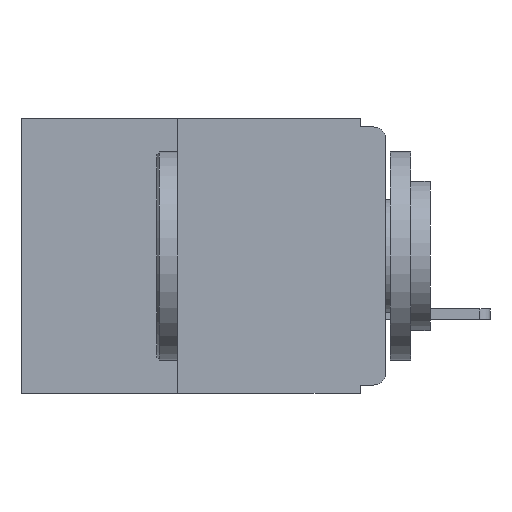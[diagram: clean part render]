
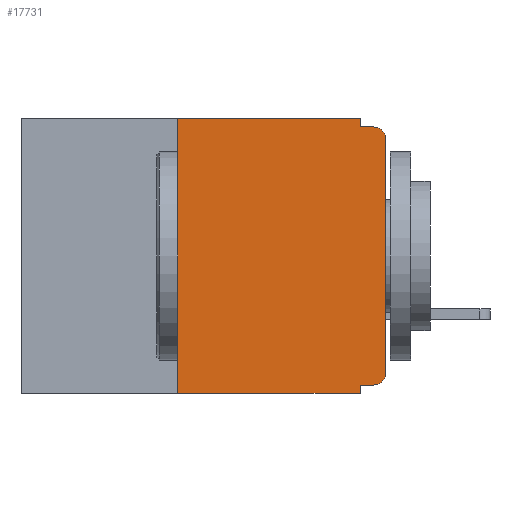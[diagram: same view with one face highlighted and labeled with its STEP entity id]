
A CAD part, left-side view. The second image highlights one B-rep face of the part: STEP entity #17731.
In plain terms, the highlighted planar face has unit normal (-1, 0, 0).
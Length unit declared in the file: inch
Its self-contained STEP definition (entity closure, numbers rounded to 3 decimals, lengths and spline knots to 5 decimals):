
#506 = CARTESIAN_POINT ( 'NONE',  ( 0., 0.031, -0.32 ) ) ;
#950 = CARTESIAN_POINT ( 'NONE',  ( 0., 0., -0.025 ) ) ;
#2074 = ORIENTED_EDGE ( 'NONE', *, *, #11409, .T. ) ;
#2745 = CARTESIAN_POINT ( 'NONE',  ( 0., 0.25, -0.33 ) ) ;
#2907 = PLANE ( 'NONE',  #11886 ) ;
#3841 = VECTOR ( 'NONE', #29928, 39.37008 ) ;
#3988 = AXIS2_PLACEMENT_3D ( 'NONE', #26032, #25995, #25987 ) ;
#4123 = DIRECTION ( 'NONE',  ( 0., -1., 0. ) ) ;
#4151 = VERTEX_POINT ( 'NONE', #20872 ) ;
#5390 = CARTESIAN_POINT ( 'NONE',  ( 0., 0.437, 0. ) ) ;
#5540 = CARTESIAN_POINT ( 'NONE',  ( 0., 0.25, -0.33 ) ) ;
#6380 = ORIENTED_EDGE ( 'NONE', *, *, #17411, .F. ) ;
#6821 = LINE ( 'NONE', #16327, #14170 ) ;
#6957 = VECTOR ( 'NONE', #19518, 39.37008 ) ;
#7222 = DIRECTION ( 'NONE',  ( -1., 0., 0. ) ) ;
#8028 = EDGE_CURVE ( 'NONE', #31687, #4151, #30851, .T. ) ;
#8325 = EDGE_LOOP ( 'NONE', ( #25144, #29642, #6380, #15313, #14939, #22247, #2074, #9829, #24186, #26533 ) ) ;
#8354 = VECTOR ( 'NONE', #29744, 39.37008 ) ;
#8696 = VERTEX_POINT ( 'NONE', #15458 ) ;
#8915 = CARTESIAN_POINT ( 'NONE',  ( 0., 0.015, -0.32 ) ) ;
#9132 = VERTEX_POINT ( 'NONE', #8915 ) ;
#9829 = ORIENTED_EDGE ( 'NONE', *, *, #23511, .F. ) ;
#10170 = VERTEX_POINT ( 'NONE', #30036 ) ;
#10405 = DIRECTION ( 'NONE',  ( 0., 0., -1. ) ) ;
#10581 = DIRECTION ( 'NONE',  ( 0., 1., 0. ) ) ;
#11018 = EDGE_CURVE ( 'NONE', #27169, #8696, #6821, .T. ) ;
#11409 = EDGE_CURVE ( 'NONE', #24281, #10170, #15683, .T. ) ;
#11446 = VERTEX_POINT ( 'NONE', #506 ) ;
#11886 = AXIS2_PLACEMENT_3D ( 'NONE', #5390, #25047, #10405 ) ;
#12027 = CARTESIAN_POINT ( 'NONE',  ( 0., 0.25, 0. ) ) ;
#12152 = CARTESIAN_POINT ( 'NONE',  ( 0., 0., 0. ) ) ;
#12219 = AXIS2_PLACEMENT_3D ( 'NONE', #21939, #7222, #24392 ) ;
#13552 = LINE ( 'NONE', #12152, #6957 ) ;
#13619 = VECTOR ( 'NONE', #15026, 39.37008 ) ;
#14170 = VECTOR ( 'NONE', #30829, 39.37008 ) ;
#14939 = ORIENTED_EDGE ( 'NONE', *, *, #11018, .F. ) ;
#15026 = DIRECTION ( 'NONE',  ( 0., 0., -1. ) ) ;
#15248 = CARTESIAN_POINT ( 'NONE',  ( 0., 0.437, -0.33 ) ) ;
#15313 = ORIENTED_EDGE ( 'NONE', *, *, #31524, .F. ) ;
#15415 = FACE_OUTER_BOUND ( 'NONE', #8325, .T. ) ;
#15458 = CARTESIAN_POINT ( 'NONE',  ( 0., 0.031, 0. ) ) ;
#15683 = LINE ( 'NONE', #15248, #8354 ) ;
#15692 = VERTEX_POINT ( 'NONE', #25230 ) ;
#16327 = CARTESIAN_POINT ( 'NONE',  ( 0., 0.437, 0. ) ) ;
#16963 = LINE ( 'NONE', #25108, #3841 ) ;
#17175 = EDGE_CURVE ( 'NONE', #24281, #27169, #31350, .T. ) ;
#17411 = EDGE_CURVE ( 'NONE', #15692, #4151, #24580, .T. ) ;
#17731 = ADVANCED_FACE ( 'NONE', ( #15415 ), #2907, .F. ) ;
#17858 = CARTESIAN_POINT ( 'NONE',  ( 0., 0., -0.32 ) ) ;
#18508 = VECTOR ( 'NONE', #20308, 39.37008 ) ;
#19518 = DIRECTION ( 'NONE',  ( 0., 0., 1. ) ) ;
#20308 = DIRECTION ( 'NONE',  ( 0., 0., 1. ) ) ;
#20872 = CARTESIAN_POINT ( 'NONE',  ( 0., 0.015, -0.01 ) ) ;
#20886 = LINE ( 'NONE', #24625, #13619 ) ;
#21939 = CARTESIAN_POINT ( 'NONE',  ( 0., 0.015, -0.305 ) ) ;
#22247 = ORIENTED_EDGE ( 'NONE', *, *, #17175, .F. ) ;
#22639 = VECTOR ( 'NONE', #10581, 39.37008 ) ;
#22714 = EDGE_CURVE ( 'NONE', #26051, #31687, #13552, .T. ) ;
#23320 = EDGE_CURVE ( 'NONE', #9132, #26051, #29488, .T. ) ;
#23426 = LINE ( 'NONE', #17858, #22639 ) ;
#23511 = EDGE_CURVE ( 'NONE', #11446, #10170, #16963, .T. ) ;
#23605 = CARTESIAN_POINT ( 'NONE',  ( 0., 0., -0.01 ) ) ;
#23830 = VECTOR ( 'NONE', #4123, 39.37008 ) ;
#24186 = ORIENTED_EDGE ( 'NONE', *, *, #24347, .F. ) ;
#24281 = VERTEX_POINT ( 'NONE', #2745 ) ;
#24347 = EDGE_CURVE ( 'NONE', #9132, #11446, #23426, .T. ) ;
#24392 = DIRECTION ( 'NONE',  ( 0., 0., -1. ) ) ;
#24575 = CARTESIAN_POINT ( 'NONE',  ( 0., 0., -0.305 ) ) ;
#24580 = LINE ( 'NONE', #23605, #23830 ) ;
#24625 = CARTESIAN_POINT ( 'NONE',  ( 0., 0.031, 0. ) ) ;
#25047 = DIRECTION ( 'NONE',  ( 1., 0., 0. ) ) ;
#25108 = CARTESIAN_POINT ( 'NONE',  ( 0., 0.031, -0.33 ) ) ;
#25144 = ORIENTED_EDGE ( 'NONE', *, *, #22714, .T. ) ;
#25230 = CARTESIAN_POINT ( 'NONE',  ( 0., 0.031, -0.01 ) ) ;
#25987 = DIRECTION ( 'NONE',  ( 0., 0., -1. ) ) ;
#25995 = DIRECTION ( 'NONE',  ( -1., 0., 0. ) ) ;
#26032 = CARTESIAN_POINT ( 'NONE',  ( 0., 0.015, -0.025 ) ) ;
#26051 = VERTEX_POINT ( 'NONE', #24575 ) ;
#26533 = ORIENTED_EDGE ( 'NONE', *, *, #23320, .T. ) ;
#27169 = VERTEX_POINT ( 'NONE', #12027 ) ;
#29488 = CIRCLE ( 'NONE', #12219, 0.015 ) ;
#29642 = ORIENTED_EDGE ( 'NONE', *, *, #8028, .T. ) ;
#29744 = DIRECTION ( 'NONE',  ( 0., -1., 0. ) ) ;
#29928 = DIRECTION ( 'NONE',  ( 0., 0., -1. ) ) ;
#30036 = CARTESIAN_POINT ( 'NONE',  ( 0., 0.031, -0.33 ) ) ;
#30829 = DIRECTION ( 'NONE',  ( 0., -1., 0. ) ) ;
#30851 = CIRCLE ( 'NONE', #3988, 0.015 ) ;
#31350 = LINE ( 'NONE', #5540, #18508 ) ;
#31524 = EDGE_CURVE ( 'NONE', #8696, #15692, #20886, .T. ) ;
#31687 = VERTEX_POINT ( 'NONE', #950 ) ;
